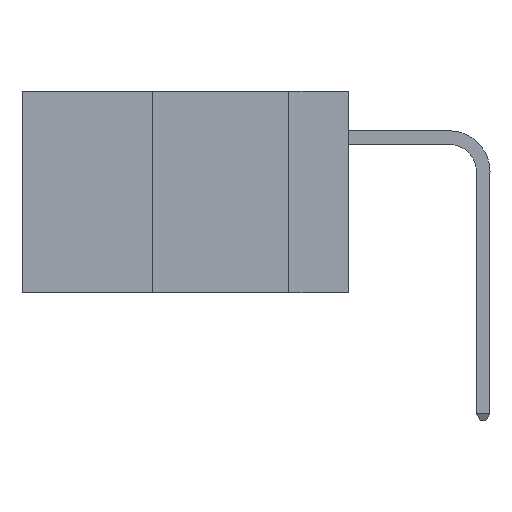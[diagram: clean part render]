
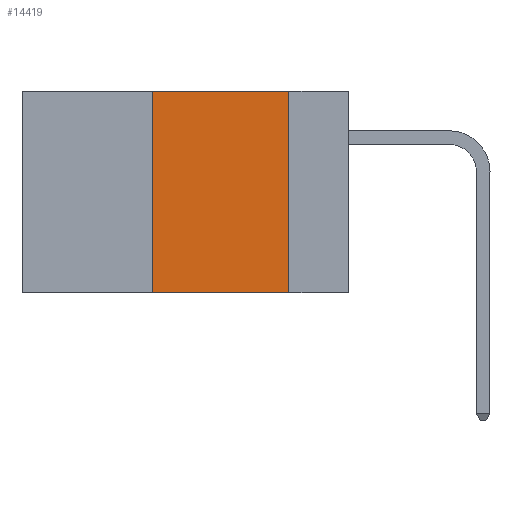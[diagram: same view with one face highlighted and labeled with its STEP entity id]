
A CAD part, left-side view. The second image highlights one B-rep face of the part: STEP entity #14419.
In plain terms, the highlighted planar face has unit normal (-1, 0, 0).
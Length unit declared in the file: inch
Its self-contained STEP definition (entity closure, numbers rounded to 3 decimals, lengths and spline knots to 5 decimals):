
#345 = EDGE_CURVE ( 'NONE', #13156, #20222, #12009, .T. ) ;
#644 = DIRECTION ( 'NONE',  ( 0., -1., 0. ) ) ;
#951 = CARTESIAN_POINT ( 'NONE',  ( 0., 0.11, 0. ) ) ;
#1176 = LINE ( 'NONE', #22074, #15228 ) ;
#2500 = CARTESIAN_POINT ( 'NONE',  ( 0., 0.36, -0.37 ) ) ;
#2654 = DIRECTION ( 'NONE',  ( 0., 0., -1. ) ) ;
#3561 = EDGE_LOOP ( 'NONE', ( #19030, #18467, #5800, #23888 ) ) ;
#5800 = ORIENTED_EDGE ( 'NONE', *, *, #7039, .F. ) ;
#5930 = CARTESIAN_POINT ( 'NONE',  ( 0., 0.6, 0. ) ) ;
#6177 = LINE ( 'NONE', #10286, #11840 ) ;
#7039 = EDGE_CURVE ( 'NONE', #19426, #9959, #20038, .T. ) ;
#7845 = DIRECTION ( 'NONE',  ( 0., 0., -1. ) ) ;
#8712 = CARTESIAN_POINT ( 'NONE',  ( 0., 0.36, 0. ) ) ;
#9677 = PLANE ( 'NONE',  #11202 ) ;
#9959 = VERTEX_POINT ( 'NONE', #10004 ) ;
#10004 = CARTESIAN_POINT ( 'NONE',  ( 0., 0.36, 0. ) ) ;
#10286 = CARTESIAN_POINT ( 'NONE',  ( 0., 0.6, -0.37 ) ) ;
#10633 = DIRECTION ( 'NONE',  ( 0., 0., 1. ) ) ;
#10888 = DIRECTION ( 'NONE',  ( 0., -1., 0. ) ) ;
#11202 = AXIS2_PLACEMENT_3D ( 'NONE', #5930, #19111, #7845 ) ;
#11840 = VECTOR ( 'NONE', #644, 39.37008 ) ;
#12009 = LINE ( 'NONE', #951, #21307 ) ;
#13156 = VERTEX_POINT ( 'NONE', #21093 ) ;
#14419 = ADVANCED_FACE ( 'NONE', ( #19124 ), #9677, .F. ) ;
#15228 = VECTOR ( 'NONE', #10888, 39.37008 ) ;
#18467 = ORIENTED_EDGE ( 'NONE', *, *, #20835, .F. ) ;
#19030 = ORIENTED_EDGE ( 'NONE', *, *, #345, .F. ) ;
#19111 = DIRECTION ( 'NONE',  ( 1., 0., 0. ) ) ;
#19124 = FACE_OUTER_BOUND ( 'NONE', #3561, .T. ) ;
#19426 = VERTEX_POINT ( 'NONE', #2500 ) ;
#19460 = VECTOR ( 'NONE', #10633, 39.37008 ) ;
#20038 = LINE ( 'NONE', #8712, #19460 ) ;
#20222 = VERTEX_POINT ( 'NONE', #21791 ) ;
#20835 = EDGE_CURVE ( 'NONE', #9959, #13156, #1176, .T. ) ;
#21093 = CARTESIAN_POINT ( 'NONE',  ( 0., 0.11, 0. ) ) ;
#21307 = VECTOR ( 'NONE', #2654, 39.37008 ) ;
#21791 = CARTESIAN_POINT ( 'NONE',  ( 0., 0.11, -0.37 ) ) ;
#22074 = CARTESIAN_POINT ( 'NONE',  ( 0., 0.6, 0. ) ) ;
#23888 = ORIENTED_EDGE ( 'NONE', *, *, #23917, .T. ) ;
#23917 = EDGE_CURVE ( 'NONE', #19426, #20222, #6177, .T. ) ;
